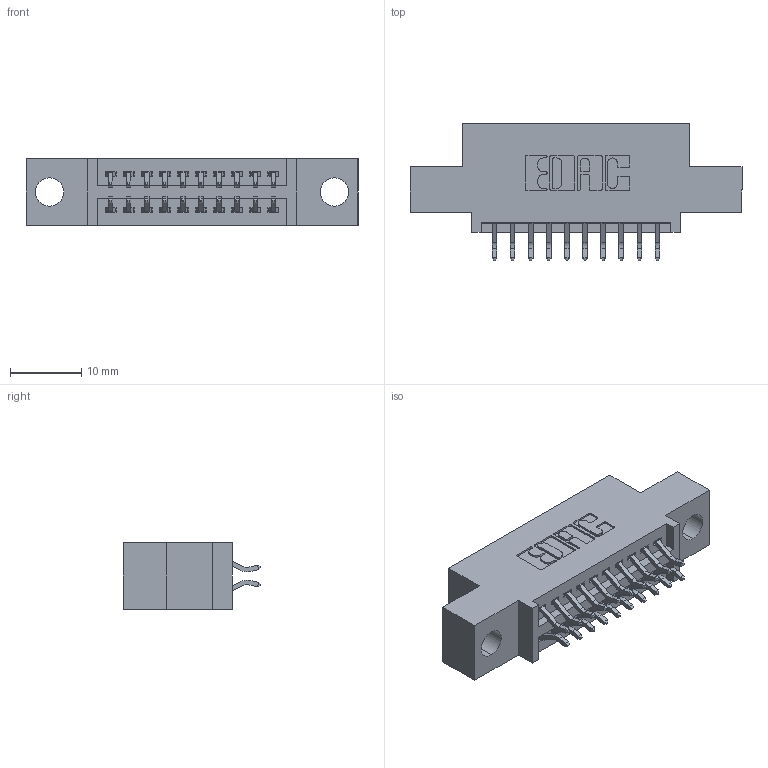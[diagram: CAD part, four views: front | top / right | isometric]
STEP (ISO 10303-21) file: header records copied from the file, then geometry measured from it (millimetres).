
FILE_DESCRIPTION (( 'STEP AP203' ), '1' );
FILE_NAME ('345-020-556-504.STEP', '2021-05-19T21:56:36', ( '' ), ( '' ), 'SwSTEP 2.0', 'SolidWorks 2020', '' );
FILE_SCHEMA (( 'CONFIG_CONTROL_DESIGN' ));
Length unit declared in the file: inch
Products named in the file (3): 345-020-556-504; 345 Part_0.110 Offset - 0.156 Dia-TI; 345-292-001_556 Tail
Assembly tree (21 placements, depth 2):
  345-020-556-504
    345 Part_0.110 Offset - 0.156 Dia-TI
    345-292-001_556 Tail  x20
Bounding box: 46.61 x 19.24 x 9.4 mm (x, y, z)
Volume: 4050.5 mm3; surface area: 5294.5 mm2
Topology: 21 solids, 21 shells, 1264 faces, 3729 edges, 2458 vertices
Faces by surface type: plane 838, cylinder 426
Entity records: 12925 total; most frequent: CARTESIAN_POINT 2218, ORIENTED_EDGE 2138, DIRECTION 1981, EDGE_CURVE 1069, VECTOR 889, LINE 889, VERTEX_POINT 710, AXIS2_PLACEMENT_3D 546
